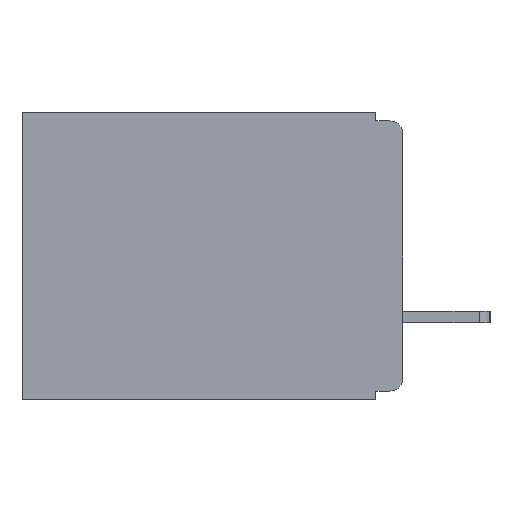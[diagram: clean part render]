
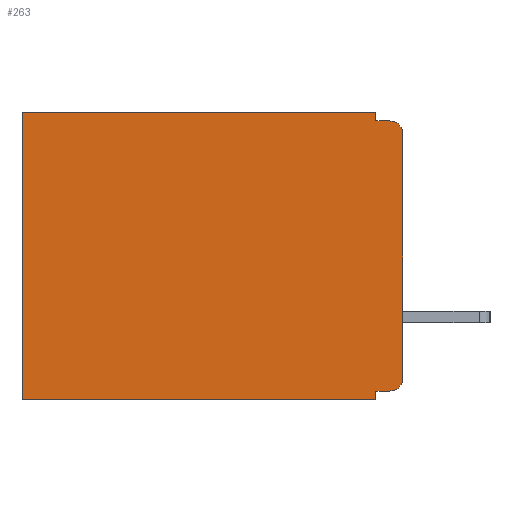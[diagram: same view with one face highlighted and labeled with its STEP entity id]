
A CAD part, left-side view. The second image highlights one B-rep face of the part: STEP entity #263.
In plain terms, the highlighted planar face has unit normal (-1, 0, 0).
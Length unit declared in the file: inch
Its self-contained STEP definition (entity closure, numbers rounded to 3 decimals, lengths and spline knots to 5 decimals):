
#16 = VERTEX_POINT ( 'NONE', #6293 ) ;
#263 = ADVANCED_FACE ( 'NONE', ( #4448 ), #6994, .F. ) ;
#415 = LINE ( 'NONE', #6688, #3325 ) ;
#486 = VERTEX_POINT ( 'NONE', #2697 ) ;
#586 = DIRECTION ( 'NONE',  ( 1., 0., 0. ) ) ;
#614 = AXIS2_PLACEMENT_3D ( 'NONE', #12214, #12226, #11735 ) ;
#691 = CARTESIAN_POINT ( 'NONE',  ( 0.3, 0.031, -0.32 ) ) ;
#946 = EDGE_CURVE ( 'NONE', #10127, #2787, #7135, .T. ) ;
#959 = ORIENTED_EDGE ( 'NONE', *, *, #13142, .F. ) ;
#1027 = DIRECTION ( 'NONE',  ( 0., 0., -1. ) ) ;
#1088 = VECTOR ( 'NONE', #7422, 39.37008 ) ;
#1642 = EDGE_CURVE ( 'NONE', #8911, #486, #10124, .T. ) ;
#1845 = VECTOR ( 'NONE', #6941, 39.37008 ) ;
#2090 = EDGE_CURVE ( 'NONE', #8264, #8911, #415, .T. ) ;
#2235 = CARTESIAN_POINT ( 'NONE',  ( 0.3, 0.031, -0.01 ) ) ;
#2697 = CARTESIAN_POINT ( 'NONE',  ( 0.3, 0.437, -0.33 ) ) ;
#2732 = LINE ( 'NONE', #4382, #5665 ) ;
#2787 = VERTEX_POINT ( 'NONE', #12678 ) ;
#2884 = EDGE_CURVE ( 'NONE', #3514, #6658, #5861, .T. ) ;
#2889 = VECTOR ( 'NONE', #6256, 39.37008 ) ;
#3069 = CARTESIAN_POINT ( 'NONE',  ( 0.3, 0., -0.33 ) ) ;
#3157 = CARTESIAN_POINT ( 'NONE',  ( 0.3, 0.015, -0.32 ) ) ;
#3325 = VECTOR ( 'NONE', #1027, 39.37008 ) ;
#3514 = VERTEX_POINT ( 'NONE', #10317 ) ;
#3521 = EDGE_CURVE ( 'NONE', #5768, #16, #8492, .T. ) ;
#4029 = CARTESIAN_POINT ( 'NONE',  ( 0.3, 0.031, 0. ) ) ;
#4382 = CARTESIAN_POINT ( 'NONE',  ( 0.3, 0.031, 0. ) ) ;
#4448 = FACE_OUTER_BOUND ( 'NONE', #4528, .T. ) ;
#4528 = EDGE_LOOP ( 'NONE', ( #10011, #7294, #9230, #959, #11035, #10604, #5788, #9734, #10039, #13234 ) ) ;
#4806 = VECTOR ( 'NONE', #12137, 39.37008 ) ;
#4842 = DIRECTION ( 'NONE',  ( 0., 0., -1. ) ) ;
#5153 = CARTESIAN_POINT ( 'NONE',  ( 0.3, 0.437, -0.33 ) ) ;
#5412 = CARTESIAN_POINT ( 'NONE',  ( 0.3, 0.031, -0.33 ) ) ;
#5520 = DIRECTION ( 'NONE',  ( 0., 0., -1. ) ) ;
#5616 = EDGE_CURVE ( 'NONE', #3514, #16, #9005, .T. ) ;
#5632 = VECTOR ( 'NONE', #13117, 39.37008 ) ;
#5665 = VECTOR ( 'NONE', #5520, 39.37008 ) ;
#5768 = VERTEX_POINT ( 'NONE', #3157 ) ;
#5788 = ORIENTED_EDGE ( 'NONE', *, *, #1642, .F. ) ;
#5796 = LINE ( 'NONE', #5153, #2889 ) ;
#5861 = CIRCLE ( 'NONE', #614, 0.015 ) ;
#6256 = DIRECTION ( 'NONE',  ( 0., 0., -1. ) ) ;
#6293 = CARTESIAN_POINT ( 'NONE',  ( 0.3, 0., -0.305 ) ) ;
#6658 = VERTEX_POINT ( 'NONE', #11516 ) ;
#6688 = CARTESIAN_POINT ( 'NONE',  ( 0.3, 0.031, -0.33 ) ) ;
#6930 = CARTESIAN_POINT ( 'NONE',  ( 0.3, 0., 0. ) ) ;
#6941 = DIRECTION ( 'NONE',  ( 0., 1., 0. ) ) ;
#6994 = PLANE ( 'NONE',  #13155 ) ;
#7066 = DIRECTION ( 'NONE',  ( 0., 0., -1. ) ) ;
#7135 = LINE ( 'NONE', #6930, #1088 ) ;
#7159 = EDGE_CURVE ( 'NONE', #5768, #8264, #13394, .T. ) ;
#7294 = ORIENTED_EDGE ( 'NONE', *, *, #2884, .T. ) ;
#7422 = DIRECTION ( 'NONE',  ( 0., 1., 0. ) ) ;
#7651 = CARTESIAN_POINT ( 'NONE',  ( 0.3, 0., -0.01 ) ) ;
#7973 = DIRECTION ( 'NONE',  ( -1., 0., 0. ) ) ;
#8264 = VERTEX_POINT ( 'NONE', #691 ) ;
#8367 = CARTESIAN_POINT ( 'NONE',  ( 0.3, 0., -0.33 ) ) ;
#8492 = CIRCLE ( 'NONE', #10979, 0.015 ) ;
#8911 = VERTEX_POINT ( 'NONE', #5412 ) ;
#9005 = LINE ( 'NONE', #8367, #5632 ) ;
#9230 = ORIENTED_EDGE ( 'NONE', *, *, #11961, .F. ) ;
#9456 = EDGE_CURVE ( 'NONE', #2787, #486, #5796, .T. ) ;
#9734 = ORIENTED_EDGE ( 'NONE', *, *, #2090, .F. ) ;
#10011 = ORIENTED_EDGE ( 'NONE', *, *, #5616, .F. ) ;
#10039 = ORIENTED_EDGE ( 'NONE', *, *, #7159, .F. ) ;
#10124 = LINE ( 'NONE', #10839, #1845 ) ;
#10127 = VERTEX_POINT ( 'NONE', #4029 ) ;
#10317 = CARTESIAN_POINT ( 'NONE',  ( 0.3, 0., -0.025 ) ) ;
#10400 = VERTEX_POINT ( 'NONE', #2235 ) ;
#10413 = VECTOR ( 'NONE', #10657, 39.37008 ) ;
#10544 = CARTESIAN_POINT ( 'NONE',  ( 0.3, 0.015, -0.305 ) ) ;
#10604 = ORIENTED_EDGE ( 'NONE', *, *, #9456, .T. ) ;
#10657 = DIRECTION ( 'NONE',  ( 0., -1., 0. ) ) ;
#10703 = LINE ( 'NONE', #7651, #10413 ) ;
#10839 = CARTESIAN_POINT ( 'NONE',  ( 0.3, 0., -0.33 ) ) ;
#10979 = AXIS2_PLACEMENT_3D ( 'NONE', #10544, #7973, #7066 ) ;
#11035 = ORIENTED_EDGE ( 'NONE', *, *, #946, .T. ) ;
#11516 = CARTESIAN_POINT ( 'NONE',  ( 0.3, 0.015, -0.01 ) ) ;
#11735 = DIRECTION ( 'NONE',  ( 0., 0., -1. ) ) ;
#11961 = EDGE_CURVE ( 'NONE', #10400, #6658, #10703, .T. ) ;
#12137 = DIRECTION ( 'NONE',  ( 0., 1., 0. ) ) ;
#12214 = CARTESIAN_POINT ( 'NONE',  ( 0.3, 0.015, -0.025 ) ) ;
#12226 = DIRECTION ( 'NONE',  ( -1., 0., 0. ) ) ;
#12678 = CARTESIAN_POINT ( 'NONE',  ( 0.3, 0.437, 0. ) ) ;
#13011 = CARTESIAN_POINT ( 'NONE',  ( 0.3, 0., -0.32 ) ) ;
#13117 = DIRECTION ( 'NONE',  ( 0., 0., -1. ) ) ;
#13142 = EDGE_CURVE ( 'NONE', #10127, #10400, #2732, .T. ) ;
#13155 = AXIS2_PLACEMENT_3D ( 'NONE', #3069, #586, #4842 ) ;
#13234 = ORIENTED_EDGE ( 'NONE', *, *, #3521, .T. ) ;
#13394 = LINE ( 'NONE', #13011, #4806 ) ;
